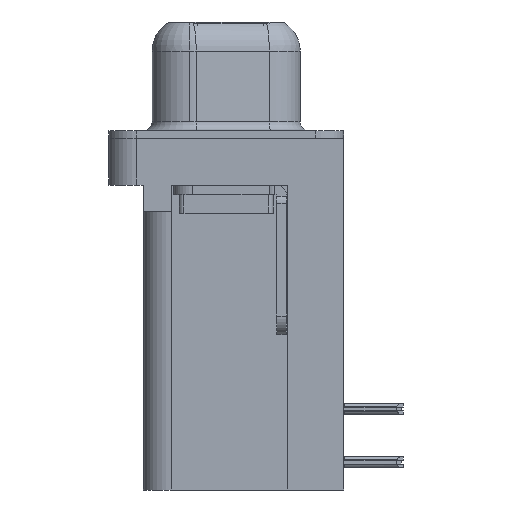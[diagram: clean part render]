
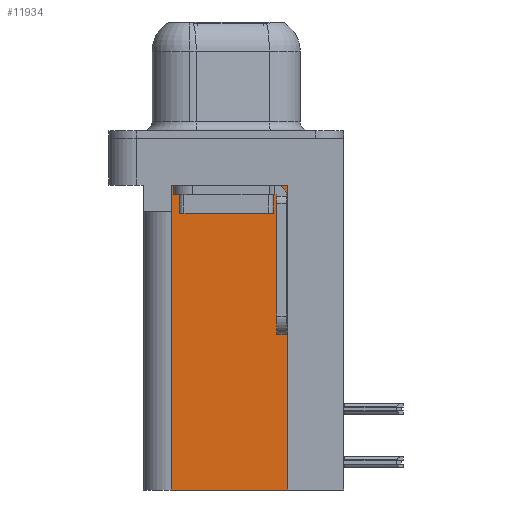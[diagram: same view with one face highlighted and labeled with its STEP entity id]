
A CAD part, left-side view. The second image highlights one B-rep face of the part: STEP entity #11934.
In plain terms, the highlighted planar face has unit normal (-1, 0, 0).
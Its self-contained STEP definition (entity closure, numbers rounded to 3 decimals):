
#175 = DIRECTION ( 'NONE',  ( 0., 1., 0. ) ) ;
#329 = VECTOR ( 'NONE', #14577, 1000. ) ;
#396 = LINE ( 'NONE', #12332, #329 ) ;
#992 = CARTESIAN_POINT ( 'NONE',  ( 3.7, -3.295, -2.5 ) ) ;
#1695 = ORIENTED_EDGE ( 'NONE', *, *, #9479, .T. ) ;
#2474 = CARTESIAN_POINT ( 'NONE',  ( 3.7, 2.925, -18.76 ) ) ;
#3410 = VECTOR ( 'NONE', #4731, 1000. ) ;
#3441 = VERTEX_POINT ( 'NONE', #4999 ) ;
#3534 = LINE ( 'NONE', #2474, #3410 ) ;
#4029 = VERTEX_POINT ( 'NONE', #22885 ) ;
#4378 = VERTEX_POINT ( 'NONE', #18238 ) ;
#4731 = DIRECTION ( 'NONE',  ( 0., 0., 1. ) ) ;
#4999 = CARTESIAN_POINT ( 'NONE',  ( 3.7, -3.295, -18.76 ) ) ;
#5518 = VERTEX_POINT ( 'NONE', #19580 ) ;
#6215 = FACE_OUTER_BOUND ( 'NONE', #23682, .T. ) ;
#6317 = CARTESIAN_POINT ( 'NONE',  ( 3.7, -3.295, -18.76 ) ) ;
#6409 = PLANE ( 'NONE',  #20757 ) ;
#6452 = DIRECTION ( 'NONE',  ( 0., 0., 1. ) ) ;
#6688 = CARTESIAN_POINT ( 'NONE',  ( 3.7, 2.895, -3.9 ) ) ;
#7418 = EDGE_CURVE ( 'NONE', #18300, #4378, #24948, .T. ) ;
#8412 = EDGE_CURVE ( 'NONE', #4378, #27434, #20531, .T. ) ;
#9479 = EDGE_CURVE ( 'NONE', #27434, #5518, #16485, .T. ) ;
#9713 = ORIENTED_EDGE ( 'NONE', *, *, #19145, .F. ) ;
#10914 = DIRECTION ( 'NONE',  ( 1., 0., 0. ) ) ;
#11190 = DIRECTION ( 'NONE',  ( 0., 0., -1. ) ) ;
#11934 = ADVANCED_FACE ( 'NONE', ( #6215 ), #6409, .F. ) ;
#12332 = CARTESIAN_POINT ( 'NONE',  ( 3.7, -3.295, -18.76 ) ) ;
#13075 = CARTESIAN_POINT ( 'NONE',  ( 3.7, 0., -3.9 ) ) ;
#14577 = DIRECTION ( 'NONE',  ( 0., 1., 0. ) ) ;
#16357 = VECTOR ( 'NONE', #17546, 1000. ) ;
#16485 = LINE ( 'NONE', #13075, #16357 ) ;
#17546 = DIRECTION ( 'NONE',  ( 0., 1., 0. ) ) ;
#17747 = ORIENTED_EDGE ( 'NONE', *, *, #20003, .F. ) ;
#18238 = CARTESIAN_POINT ( 'NONE',  ( 3.7, 2.895, -2.5 ) ) ;
#18300 = VERTEX_POINT ( 'NONE', #992 ) ;
#19145 = EDGE_CURVE ( 'NONE', #4029, #5518, #3534, .T. ) ;
#19580 = CARTESIAN_POINT ( 'NONE',  ( 3.7, 2.925, -3.9 ) ) ;
#20003 = EDGE_CURVE ( 'NONE', #3441, #4029, #396, .T. ) ;
#20072 = VECTOR ( 'NONE', #6452, 1000. ) ;
#20261 = EDGE_CURVE ( 'NONE', #3441, #18300, #27874, .T. ) ;
#20509 = VECTOR ( 'NONE', #11190, 1000. ) ;
#20531 = LINE ( 'NONE', #6688, #20509 ) ;
#20757 = AXIS2_PLACEMENT_3D ( 'NONE', #6317, #10914, #26233 ) ;
#21909 = CARTESIAN_POINT ( 'NONE',  ( 3.7, -3.295, -18.76 ) ) ;
#22885 = CARTESIAN_POINT ( 'NONE',  ( 3.7, 2.925, -18.76 ) ) ;
#22940 = CARTESIAN_POINT ( 'NONE',  ( 3.7, 2.895, -3.9 ) ) ;
#23682 = EDGE_LOOP ( 'NONE', ( #26434, #25909, #1695, #9713, #17747, #26204 ) ) ;
#24750 = VECTOR ( 'NONE', #175, 1000. ) ;
#24948 = LINE ( 'NONE', #26659, #24750 ) ;
#25909 = ORIENTED_EDGE ( 'NONE', *, *, #8412, .T. ) ;
#26204 = ORIENTED_EDGE ( 'NONE', *, *, #20261, .T. ) ;
#26233 = DIRECTION ( 'NONE',  ( 0., 1., 0. ) ) ;
#26434 = ORIENTED_EDGE ( 'NONE', *, *, #7418, .T. ) ;
#26659 = CARTESIAN_POINT ( 'NONE',  ( 3.7, -3.295, -2.5 ) ) ;
#27434 = VERTEX_POINT ( 'NONE', #22940 ) ;
#27874 = LINE ( 'NONE', #21909, #20072 ) ;
